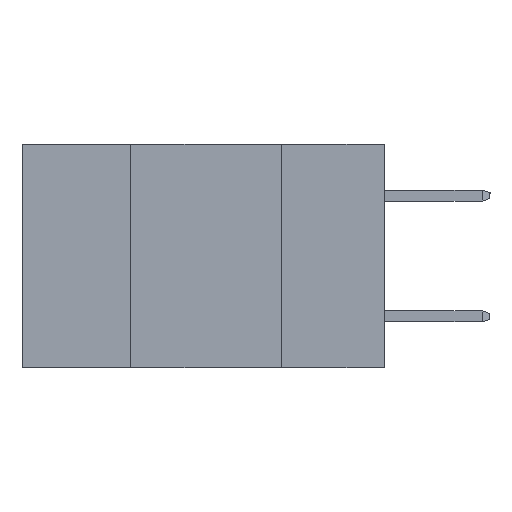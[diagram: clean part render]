
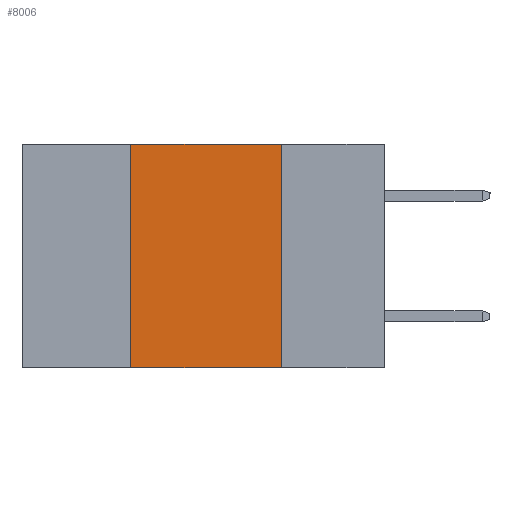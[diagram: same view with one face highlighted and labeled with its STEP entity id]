
A CAD part, left-side view. The second image highlights one B-rep face of the part: STEP entity #8006.
In plain terms, the highlighted planar face has unit normal (-1, 0, 0).
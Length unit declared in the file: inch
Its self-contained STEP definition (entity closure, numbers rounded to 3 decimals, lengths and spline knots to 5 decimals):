
#469 = CARTESIAN_POINT ( 'NONE',  ( 0., 0.6, 0. ) ) ;
#1156 = CARTESIAN_POINT ( 'NONE',  ( 0., 0.6, 0. ) ) ;
#1443 = VERTEX_POINT ( 'NONE', #4497 ) ;
#1842 = ORIENTED_EDGE ( 'NONE', *, *, #8680, .F. ) ;
#1995 = ORIENTED_EDGE ( 'NONE', *, *, #3355, .F. ) ;
#2473 = LINE ( 'NONE', #8126, #9098 ) ;
#2546 = CARTESIAN_POINT ( 'NONE',  ( 0., 0.6, -0.37 ) ) ;
#2723 = DIRECTION ( 'NONE',  ( 0., 0., -1. ) ) ;
#2897 = VECTOR ( 'NONE', #8069, 39.37008 ) ;
#3355 = EDGE_CURVE ( 'NONE', #9207, #1443, #10186, .T. ) ;
#3711 = EDGE_CURVE ( 'NONE', #1443, #6475, #2473, .T. ) ;
#4067 = CARTESIAN_POINT ( 'NONE',  ( 0., 0.17, -0.37 ) ) ;
#4497 = CARTESIAN_POINT ( 'NONE',  ( 0., 0.17, 0. ) ) ;
#4920 = LINE ( 'NONE', #2546, #7629 ) ;
#5006 = VERTEX_POINT ( 'NONE', #6955 ) ;
#5231 = PLANE ( 'NONE',  #5925 ) ;
#5819 = ORIENTED_EDGE ( 'NONE', *, *, #9046, .T. ) ;
#5925 = AXIS2_PLACEMENT_3D ( 'NONE', #469, #6132, #9942 ) ;
#6132 = DIRECTION ( 'NONE',  ( 1., 0., 0. ) ) ;
#6307 = EDGE_LOOP ( 'NONE', ( #9251, #1995, #1842, #5819 ) ) ;
#6375 = CARTESIAN_POINT ( 'NONE',  ( 0., 0.42, -0.37 ) ) ;
#6475 = VERTEX_POINT ( 'NONE', #4067 ) ;
#6878 = FACE_OUTER_BOUND ( 'NONE', #6307, .T. ) ;
#6955 = CARTESIAN_POINT ( 'NONE',  ( 0., 0.42, -0.37 ) ) ;
#7240 = VECTOR ( 'NONE', #9244, 39.37008 ) ;
#7432 = LINE ( 'NONE', #6375, #2897 ) ;
#7629 = VECTOR ( 'NONE', #9003, 39.37008 ) ;
#8006 = ADVANCED_FACE ( 'NONE', ( #6878 ), #5231, .F. ) ;
#8069 = DIRECTION ( 'NONE',  ( 0., 0., 1. ) ) ;
#8126 = CARTESIAN_POINT ( 'NONE',  ( 0., 0.17, -0.37 ) ) ;
#8680 = EDGE_CURVE ( 'NONE', #5006, #9207, #7432, .T. ) ;
#9003 = DIRECTION ( 'NONE',  ( 0., -1., 0. ) ) ;
#9046 = EDGE_CURVE ( 'NONE', #5006, #6475, #4920, .T. ) ;
#9098 = VECTOR ( 'NONE', #2723, 39.37008 ) ;
#9207 = VERTEX_POINT ( 'NONE', #9354 ) ;
#9244 = DIRECTION ( 'NONE',  ( 0., -1., 0. ) ) ;
#9251 = ORIENTED_EDGE ( 'NONE', *, *, #3711, .F. ) ;
#9354 = CARTESIAN_POINT ( 'NONE',  ( 0., 0.42, 0. ) ) ;
#9942 = DIRECTION ( 'NONE',  ( 0., 0., -1. ) ) ;
#10186 = LINE ( 'NONE', #1156, #7240 ) ;
